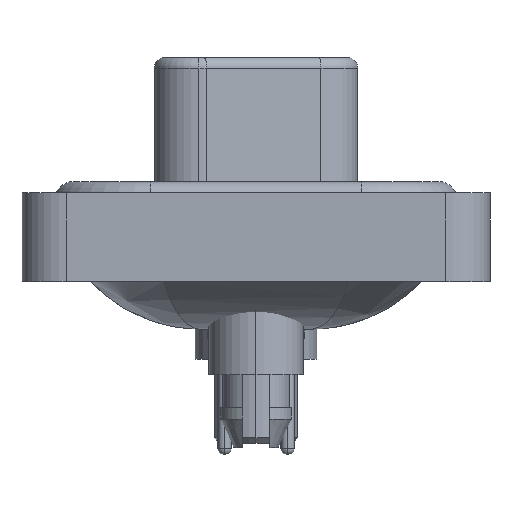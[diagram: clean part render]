
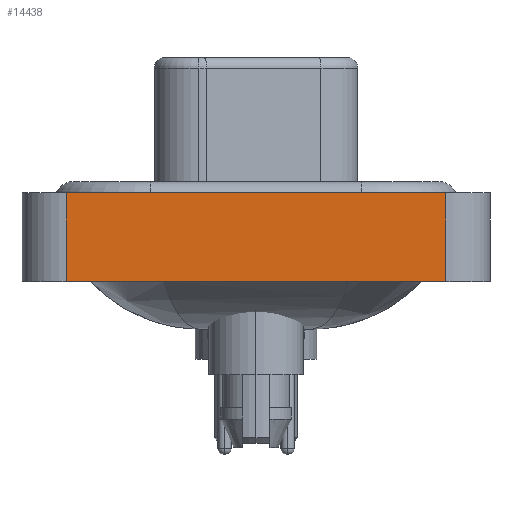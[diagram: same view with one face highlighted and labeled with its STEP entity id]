
A CAD part, left-side view. The second image highlights one B-rep face of the part: STEP entity #14438.
In plain terms, the highlighted planar face has unit normal (-1, 0, 0).
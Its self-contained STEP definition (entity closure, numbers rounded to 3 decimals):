
#2971 = CARTESIAN_POINT ( 'NONE',  ( -7.3, -8.55, -3.6 ) ) ;
#3063 = EDGE_CURVE ( 'NONE', #9570, #17828, #21382, .T. ) ;
#4121 = VECTOR ( 'NONE', #13070, 1000. ) ;
#4904 = VERTEX_POINT ( 'NONE', #7039 ) ;
#4951 = EDGE_CURVE ( 'NONE', #4904, #9570, #17941, .T. ) ;
#6951 = DIRECTION ( 'NONE',  ( -1., 0., 0. ) ) ;
#7039 = CARTESIAN_POINT ( 'NONE',  ( -7.3, 8.55, -3.6 ) ) ;
#7654 = VECTOR ( 'NONE', #11247, 1000. ) ;
#7833 = VECTOR ( 'NONE', #9951, 1000. ) ;
#8487 = DIRECTION ( 'NONE',  ( 0., 0., 1. ) ) ;
#8928 = CARTESIAN_POINT ( 'NONE',  ( -7.3, -8.55, -3.6 ) ) ;
#9066 = AXIS2_PLACEMENT_3D ( 'NONE', #8928, #6951, #8487 ) ;
#9341 = CARTESIAN_POINT ( 'NONE',  ( -7.3, 8.55, -3.6 ) ) ;
#9496 = EDGE_LOOP ( 'NONE', ( #13474, #15216, #14364, #13641 ) ) ;
#9570 = VERTEX_POINT ( 'NONE', #20805 ) ;
#9745 = CARTESIAN_POINT ( 'NONE',  ( -7.3, -8.55, -3.6 ) ) ;
#9951 = DIRECTION ( 'NONE',  ( 0., 0., 1. ) ) ;
#11247 = DIRECTION ( 'NONE',  ( 0., -1., 0. ) ) ;
#11359 = CARTESIAN_POINT ( 'NONE',  ( -7.3, -8.55, -3.6 ) ) ;
#13070 = DIRECTION ( 'NONE',  ( 0., -1., 0. ) ) ;
#13246 = CARTESIAN_POINT ( 'NONE',  ( -7.3, -8.55, 0.4 ) ) ;
#13474 = ORIENTED_EDGE ( 'NONE', *, *, #20409, .T. ) ;
#13641 = ORIENTED_EDGE ( 'NONE', *, *, #14060, .T. ) ;
#14060 = EDGE_CURVE ( 'NONE', #4904, #19076, #14074, .T. ) ;
#14074 = LINE ( 'NONE', #2971, #7654 ) ;
#14364 = ORIENTED_EDGE ( 'NONE', *, *, #4951, .F. ) ;
#14438 = ADVANCED_FACE ( 'NONE', ( #16995 ), #20500, .T. ) ;
#15216 = ORIENTED_EDGE ( 'NONE', *, *, #3063, .F. ) ;
#16995 = FACE_OUTER_BOUND ( 'NONE', #9496, .T. ) ;
#17657 = VECTOR ( 'NONE', #19474, 1000. ) ;
#17828 = VERTEX_POINT ( 'NONE', #13246 ) ;
#17941 = LINE ( 'NONE', #9341, #17657 ) ;
#18025 = LINE ( 'NONE', #9745, #7833 ) ;
#19076 = VERTEX_POINT ( 'NONE', #11359 ) ;
#19474 = DIRECTION ( 'NONE',  ( 0., 0., 1. ) ) ;
#19616 = CARTESIAN_POINT ( 'NONE',  ( -7.3, -8.55, 0.4 ) ) ;
#20409 = EDGE_CURVE ( 'NONE', #19076, #17828, #18025, .T. ) ;
#20500 = PLANE ( 'NONE',  #9066 ) ;
#20805 = CARTESIAN_POINT ( 'NONE',  ( -7.3, 8.55, 0.4 ) ) ;
#21382 = LINE ( 'NONE', #19616, #4121 ) ;
